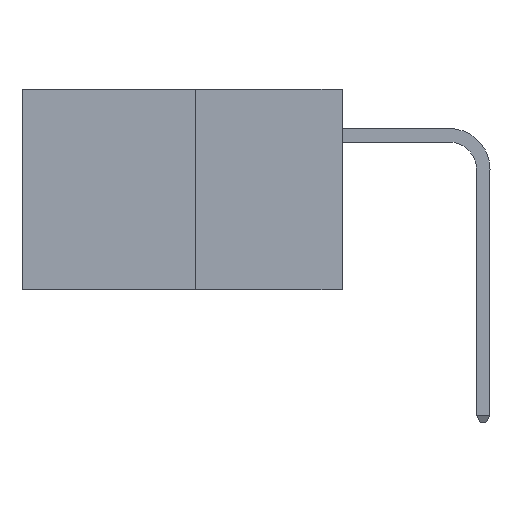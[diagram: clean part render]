
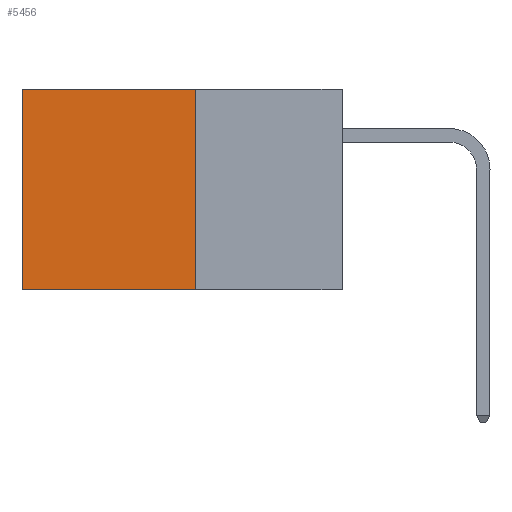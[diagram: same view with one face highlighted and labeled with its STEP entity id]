
A CAD part, left-side view. The second image highlights one B-rep face of the part: STEP entity #5456.
In plain terms, the highlighted planar face has unit normal (-1, 0, 0).
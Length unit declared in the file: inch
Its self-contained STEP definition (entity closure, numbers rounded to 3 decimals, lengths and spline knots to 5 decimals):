
#1162 = AXIS2_PLACEMENT_3D ( 'NONE', #8638, #8667, #8519 ) ;
#1410 = VECTOR ( 'NONE', #7345, 39.37008 ) ;
#1885 = LINE ( 'NONE', #20402, #19654 ) ;
#3540 = EDGE_CURVE ( 'NONE', #6921, #21226, #5783, .T. ) ;
#4190 = VECTOR ( 'NONE', #21813, 39.37008 ) ;
#4295 = CARTESIAN_POINT ( 'NONE',  ( 0.277, 0.27, 0. ) ) ;
#5456 = ADVANCED_FACE ( 'NONE', ( #8207 ), #6678, .F. ) ;
#5783 = LINE ( 'NONE', #16338, #10463 ) ;
#6150 = LINE ( 'NONE', #7712, #1410 ) ;
#6678 = PLANE ( 'NONE',  #1162 ) ;
#6921 = VERTEX_POINT ( 'NONE', #4295 ) ;
#7229 = DIRECTION ( 'NONE',  ( 0., 0., -1. ) ) ;
#7240 = ORIENTED_EDGE ( 'NONE', *, *, #3540, .F. ) ;
#7345 = DIRECTION ( 'NONE',  ( 0., 1., 0. ) ) ;
#7398 = EDGE_LOOP ( 'NONE', ( #9088, #17046, #7240, #21979 ) ) ;
#7712 = CARTESIAN_POINT ( 'NONE',  ( 0.277, 0.27, -0.37 ) ) ;
#8094 = CARTESIAN_POINT ( 'NONE',  ( 0.277, 0.27, -0.37 ) ) ;
#8207 = FACE_OUTER_BOUND ( 'NONE', #7398, .T. ) ;
#8241 = EDGE_CURVE ( 'NONE', #21226, #15620, #6150, .T. ) ;
#8496 = CARTESIAN_POINT ( 'NONE',  ( 0.277, 0.59, 0. ) ) ;
#8519 = DIRECTION ( 'NONE',  ( 0., 0., -1. ) ) ;
#8638 = CARTESIAN_POINT ( 'NONE',  ( 0.277, 0.27, -0.37 ) ) ;
#8667 = DIRECTION ( 'NONE',  ( 1., 0., 0. ) ) ;
#8782 = CARTESIAN_POINT ( 'NONE',  ( 0.277, 0.59, -0.37 ) ) ;
#9088 = ORIENTED_EDGE ( 'NONE', *, *, #9470, .T. ) ;
#9470 = EDGE_CURVE ( 'NONE', #18072, #15620, #1885, .T. ) ;
#10463 = VECTOR ( 'NONE', #7229, 39.37008 ) ;
#13498 = CARTESIAN_POINT ( 'NONE',  ( 0.277, 0.27, 0. ) ) ;
#15620 = VERTEX_POINT ( 'NONE', #8782 ) ;
#16338 = CARTESIAN_POINT ( 'NONE',  ( 0.277, 0.27, -0.37 ) ) ;
#17046 = ORIENTED_EDGE ( 'NONE', *, *, #8241, .F. ) ;
#17414 = LINE ( 'NONE', #13498, #4190 ) ;
#18072 = VERTEX_POINT ( 'NONE', #8496 ) ;
#18686 = EDGE_CURVE ( 'NONE', #6921, #18072, #17414, .T. ) ;
#19654 = VECTOR ( 'NONE', #21335, 39.37008 ) ;
#20402 = CARTESIAN_POINT ( 'NONE',  ( 0.277, 0.59, -0.37 ) ) ;
#21226 = VERTEX_POINT ( 'NONE', #8094 ) ;
#21335 = DIRECTION ( 'NONE',  ( 0., 0., -1. ) ) ;
#21813 = DIRECTION ( 'NONE',  ( 0., 1., 0. ) ) ;
#21979 = ORIENTED_EDGE ( 'NONE', *, *, #18686, .T. ) ;
